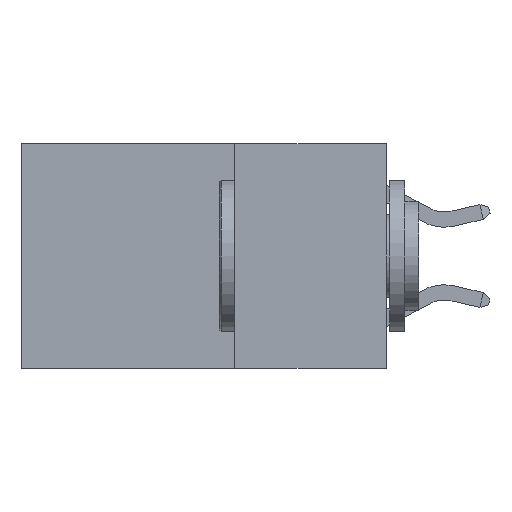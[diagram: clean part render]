
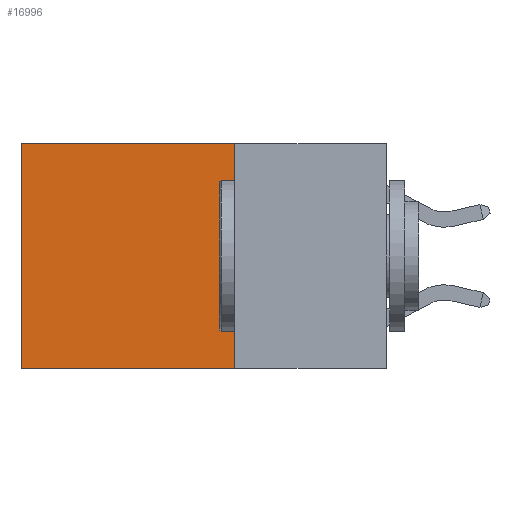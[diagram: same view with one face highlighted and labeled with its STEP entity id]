
A CAD part, left-side view. The second image highlights one B-rep face of the part: STEP entity #16996.
In plain terms, the highlighted planar face has unit normal (-1, 0, 0).
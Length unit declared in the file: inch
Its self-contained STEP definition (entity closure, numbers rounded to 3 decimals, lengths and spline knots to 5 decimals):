
#1237 = EDGE_LOOP ( 'NONE', ( #10039, #13793, #4391, #4437 ) ) ;
#2710 = CARTESIAN_POINT ( 'NONE',  ( 0.2625, 0.25, 0. ) ) ;
#3286 = CARTESIAN_POINT ( 'NONE',  ( 0.2625, 0.25, 0. ) ) ;
#4181 = CARTESIAN_POINT ( 'NONE',  ( 0.2625, 0.6, -0.37 ) ) ;
#4287 = CARTESIAN_POINT ( 'NONE',  ( 0.2625, 0.25, -0.37 ) ) ;
#4391 = ORIENTED_EDGE ( 'NONE', *, *, #19192, .F. ) ;
#4437 = ORIENTED_EDGE ( 'NONE', *, *, #21936, .T. ) ;
#6209 = VERTEX_POINT ( 'NONE', #13616 ) ;
#7399 = PLANE ( 'NONE',  #15710 ) ;
#7434 = CARTESIAN_POINT ( 'NONE',  ( 0.2625, 0.25, -0.37 ) ) ;
#7488 = CARTESIAN_POINT ( 'NONE',  ( 0.2625, 0.25, 0. ) ) ;
#8205 = VECTOR ( 'NONE', #17552, 39.37008 ) ;
#8486 = VERTEX_POINT ( 'NONE', #4181 ) ;
#8785 = EDGE_CURVE ( 'NONE', #16970, #8486, #22428, .T. ) ;
#10039 = ORIENTED_EDGE ( 'NONE', *, *, #8785, .T. ) ;
#10389 = VECTOR ( 'NONE', #24729, 39.37008 ) ;
#11447 = FACE_OUTER_BOUND ( 'NONE', #1237, .T. ) ;
#12281 = LINE ( 'NONE', #7434, #8205 ) ;
#12966 = EDGE_CURVE ( 'NONE', #19817, #8486, #12281, .T. ) ;
#13030 = CARTESIAN_POINT ( 'NONE',  ( 0.2625, 0.6, 0. ) ) ;
#13476 = DIRECTION ( 'NONE',  ( 0., 0., -1. ) ) ;
#13616 = CARTESIAN_POINT ( 'NONE',  ( 0.2625, 0.25, 0. ) ) ;
#13793 = ORIENTED_EDGE ( 'NONE', *, *, #12966, .F. ) ;
#15620 = DIRECTION ( 'NONE',  ( 0., 0., -1. ) ) ;
#15710 = AXIS2_PLACEMENT_3D ( 'NONE', #7488, #23337, #13476 ) ;
#16970 = VERTEX_POINT ( 'NONE', #13030 ) ;
#16996 = ADVANCED_FACE ( 'NONE', ( #11447 ), #7399, .F. ) ;
#17552 = DIRECTION ( 'NONE',  ( 0., 1., 0. ) ) ;
#18346 = VECTOR ( 'NONE', #15620, 39.37008 ) ;
#18577 = CARTESIAN_POINT ( 'NONE',  ( 0.2625, 0.6, 0. ) ) ;
#19192 = EDGE_CURVE ( 'NONE', #6209, #19817, #19291, .T. ) ;
#19291 = LINE ( 'NONE', #3286, #18346 ) ;
#19817 = VERTEX_POINT ( 'NONE', #4287 ) ;
#20503 = DIRECTION ( 'NONE',  ( 0., 0., -1. ) ) ;
#20560 = VECTOR ( 'NONE', #20503, 39.37008 ) ;
#21936 = EDGE_CURVE ( 'NONE', #6209, #16970, #22492, .T. ) ;
#22428 = LINE ( 'NONE', #18577, #20560 ) ;
#22492 = LINE ( 'NONE', #2710, #10389 ) ;
#23337 = DIRECTION ( 'NONE',  ( 1., 0., 0. ) ) ;
#24729 = DIRECTION ( 'NONE',  ( 0., 1., 0. ) ) ;
